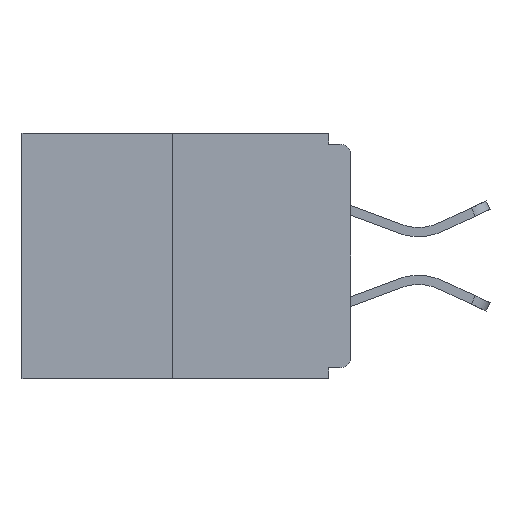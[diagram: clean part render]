
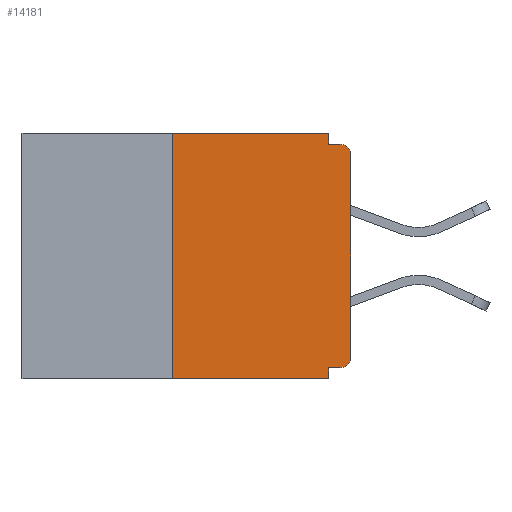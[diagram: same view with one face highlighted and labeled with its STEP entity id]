
A CAD part, left-side view. The second image highlights one B-rep face of the part: STEP entity #14181.
In plain terms, the highlighted planar face has unit normal (-1, 0, 0).
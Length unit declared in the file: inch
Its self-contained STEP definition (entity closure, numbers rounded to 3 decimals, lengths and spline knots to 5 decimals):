
#692 = CARTESIAN_POINT ( 'NONE',  ( 0., 0.031, -0.015 ) ) ;
#847 = VECTOR ( 'NONE', #18085, 39.37008 ) ;
#1480 = CARTESIAN_POINT ( 'NONE',  ( 0., 0.031, 0. ) ) ;
#1530 = VERTEX_POINT ( 'NONE', #3660 ) ;
#1590 = EDGE_CURVE ( 'NONE', #1530, #28177, #2432, .T. ) ;
#1819 = AXIS2_PLACEMENT_3D ( 'NONE', #27757, #23305, #19182 ) ;
#2432 = LINE ( 'NONE', #6940, #13889 ) ;
#2868 = ORIENTED_EDGE ( 'NONE', *, *, #6302, .F. ) ;
#2884 = CARTESIAN_POINT ( 'NONE',  ( 0., 0.031, -0.328 ) ) ;
#3253 = DIRECTION ( 'NONE',  ( 0., 0., -1. ) ) ;
#3521 = EDGE_CURVE ( 'NONE', #4267, #1530, #16621, .T. ) ;
#3543 = DIRECTION ( 'NONE',  ( 0., 0., -1. ) ) ;
#3660 = CARTESIAN_POINT ( 'NONE',  ( 0., 0., -0.313 ) ) ;
#4143 = CARTESIAN_POINT ( 'NONE',  ( 0., 0.031, 0. ) ) ;
#4267 = VERTEX_POINT ( 'NONE', #22345 ) ;
#4336 = LINE ( 'NONE', #6361, #847 ) ;
#4712 = CARTESIAN_POINT ( 'NONE',  ( 0., 0.031, -0.343 ) ) ;
#5154 = EDGE_CURVE ( 'NONE', #4267, #26555, #4336, .T. ) ;
#5310 = VECTOR ( 'NONE', #16424, 39.37008 ) ;
#6111 = ORIENTED_EDGE ( 'NONE', *, *, #27214, .T. ) ;
#6302 = EDGE_CURVE ( 'NONE', #17976, #23392, #26215, .T. ) ;
#6361 = CARTESIAN_POINT ( 'NONE',  ( 0., 0., -0.328 ) ) ;
#6940 = CARTESIAN_POINT ( 'NONE',  ( 0., 0., 0. ) ) ;
#7345 = LINE ( 'NONE', #8866, #12586 ) ;
#7815 = DIRECTION ( 'NONE',  ( -1., 0., 0. ) ) ;
#8022 = CARTESIAN_POINT ( 'NONE',  ( 0., 0.25, 0. ) ) ;
#8866 = CARTESIAN_POINT ( 'NONE',  ( 0., 0.46, 0. ) ) ;
#9195 = DIRECTION ( 'NONE',  ( 0., 0., 1. ) ) ;
#9804 = EDGE_LOOP ( 'NONE', ( #20706, #16882, #6111, #12900, #13928, #26096, #28818, #17842, #2868, #20848 ) ) ;
#10242 = VERTEX_POINT ( 'NONE', #4712 ) ;
#10532 = VECTOR ( 'NONE', #3543, 39.37008 ) ;
#10835 = LINE ( 'NONE', #4143, #12236 ) ;
#10882 = EDGE_CURVE ( 'NONE', #26320, #17976, #10835, .T. ) ;
#11245 = VERTEX_POINT ( 'NONE', #8022 ) ;
#11882 = AXIS2_PLACEMENT_3D ( 'NONE', #16572, #14630, #3253 ) ;
#11949 = CARTESIAN_POINT ( 'NONE',  ( 0., 0.25, 0. ) ) ;
#12236 = VECTOR ( 'NONE', #23992, 39.37008 ) ;
#12586 = VECTOR ( 'NONE', #15762, 39.37008 ) ;
#12645 = EDGE_CURVE ( 'NONE', #26882, #11245, #22239, .T. ) ;
#12900 = ORIENTED_EDGE ( 'NONE', *, *, #25974, .F. ) ;
#13889 = VECTOR ( 'NONE', #9195, 39.37008 ) ;
#13928 = ORIENTED_EDGE ( 'NONE', *, *, #5154, .F. ) ;
#14181 = ADVANCED_FACE ( 'NONE', ( #18167 ), #18401, .F. ) ;
#14516 = CARTESIAN_POINT ( 'NONE',  ( 0., 0.015, -0.313 ) ) ;
#14630 = DIRECTION ( 'NONE',  ( -1., 0., 0. ) ) ;
#14649 = CARTESIAN_POINT ( 'NONE',  ( 0., 0.015, -0.015 ) ) ;
#14863 = EDGE_CURVE ( 'NONE', #28177, #23392, #20981, .T. ) ;
#15762 = DIRECTION ( 'NONE',  ( 0., -1., 0. ) ) ;
#15815 = CARTESIAN_POINT ( 'NONE',  ( 0., 0., -0.03 ) ) ;
#16137 = AXIS2_PLACEMENT_3D ( 'NONE', #14516, #7815, #18784 ) ;
#16424 = DIRECTION ( 'NONE',  ( 0., -1., 0. ) ) ;
#16572 = CARTESIAN_POINT ( 'NONE',  ( 0., 0.015, -0.03 ) ) ;
#16621 = CIRCLE ( 'NONE', #16137, 0.015 ) ;
#16882 = ORIENTED_EDGE ( 'NONE', *, *, #12645, .F. ) ;
#17842 = ORIENTED_EDGE ( 'NONE', *, *, #14863, .T. ) ;
#17976 = VERTEX_POINT ( 'NONE', #692 ) ;
#18085 = DIRECTION ( 'NONE',  ( 0., 1., 0. ) ) ;
#18167 = FACE_OUTER_BOUND ( 'NONE', #9804, .T. ) ;
#18401 = PLANE ( 'NONE',  #1819 ) ;
#18784 = DIRECTION ( 'NONE',  ( 0., 0., -1. ) ) ;
#18858 = DIRECTION ( 'NONE',  ( 0., 0., 1. ) ) ;
#19083 = VECTOR ( 'NONE', #18858, 39.37008 ) ;
#19182 = DIRECTION ( 'NONE',  ( 0., 0., -1. ) ) ;
#20706 = ORIENTED_EDGE ( 'NONE', *, *, #24174, .F. ) ;
#20848 = ORIENTED_EDGE ( 'NONE', *, *, #10882, .F. ) ;
#20962 = LINE ( 'NONE', #21724, #10532 ) ;
#20981 = CIRCLE ( 'NONE', #11882, 0.015 ) ;
#21484 = CARTESIAN_POINT ( 'NONE',  ( 0., 0.46, -0.343 ) ) ;
#21724 = CARTESIAN_POINT ( 'NONE',  ( 0., 0.031, -0.343 ) ) ;
#22239 = LINE ( 'NONE', #11949, #19083 ) ;
#22345 = CARTESIAN_POINT ( 'NONE',  ( 0., 0.015, -0.328 ) ) ;
#23305 = DIRECTION ( 'NONE',  ( 1., 0., 0. ) ) ;
#23392 = VERTEX_POINT ( 'NONE', #14649 ) ;
#23992 = DIRECTION ( 'NONE',  ( 0., 0., -1. ) ) ;
#24174 = EDGE_CURVE ( 'NONE', #11245, #26320, #7345, .T. ) ;
#24233 = DIRECTION ( 'NONE',  ( 0., -1., 0. ) ) ;
#24399 = LINE ( 'NONE', #21484, #27473 ) ;
#25281 = CARTESIAN_POINT ( 'NONE',  ( 0., 0.25, -0.343 ) ) ;
#25480 = CARTESIAN_POINT ( 'NONE',  ( 0., 0., -0.015 ) ) ;
#25974 = EDGE_CURVE ( 'NONE', #26555, #10242, #20962, .T. ) ;
#26096 = ORIENTED_EDGE ( 'NONE', *, *, #3521, .T. ) ;
#26215 = LINE ( 'NONE', #25480, #5310 ) ;
#26320 = VERTEX_POINT ( 'NONE', #1480 ) ;
#26555 = VERTEX_POINT ( 'NONE', #2884 ) ;
#26882 = VERTEX_POINT ( 'NONE', #25281 ) ;
#27214 = EDGE_CURVE ( 'NONE', #26882, #10242, #24399, .T. ) ;
#27473 = VECTOR ( 'NONE', #24233, 39.37008 ) ;
#27757 = CARTESIAN_POINT ( 'NONE',  ( 0., 0.46, 0. ) ) ;
#28177 = VERTEX_POINT ( 'NONE', #15815 ) ;
#28818 = ORIENTED_EDGE ( 'NONE', *, *, #1590, .T. ) ;
